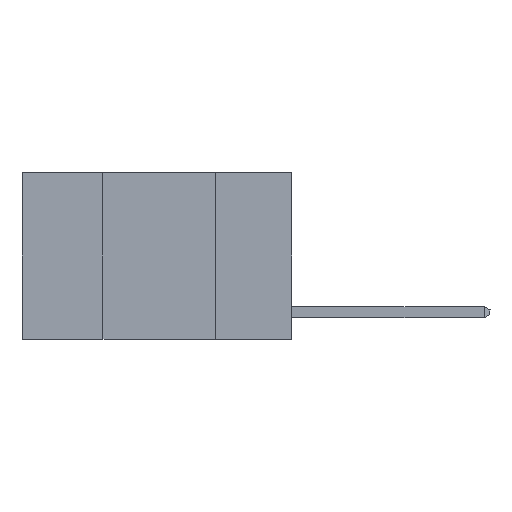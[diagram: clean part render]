
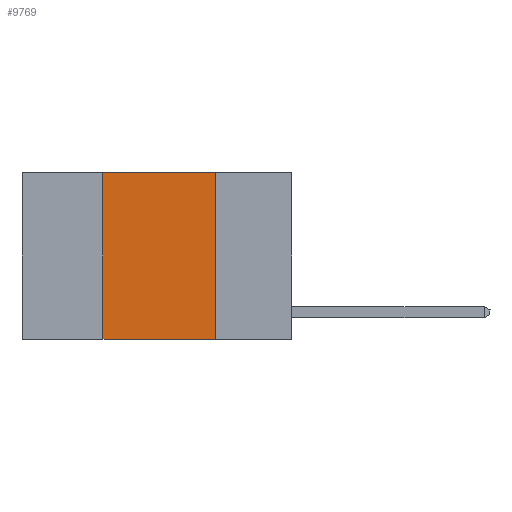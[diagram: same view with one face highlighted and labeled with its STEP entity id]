
A CAD part, left-side view. The second image highlights one B-rep face of the part: STEP entity #9769.
In plain terms, the highlighted planar face has unit normal (-1, 0, 0).
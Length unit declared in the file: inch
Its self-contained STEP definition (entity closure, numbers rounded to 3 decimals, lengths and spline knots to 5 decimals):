
#273 = LINE ( 'NONE', #14539, #352 ) ;
#352 = VECTOR ( 'NONE', #3297, 39.37008 ) ;
#1255 = ORIENTED_EDGE ( 'NONE', *, *, #9447, .F. ) ;
#1514 = VECTOR ( 'NONE', #4115, 39.37008 ) ;
#1585 = VERTEX_POINT ( 'NONE', #7413 ) ;
#3297 = DIRECTION ( 'NONE',  ( 0., -1., 0. ) ) ;
#3979 = DIRECTION ( 'NONE',  ( 0., 0., -1. ) ) ;
#3998 = LINE ( 'NONE', #9761, #4417 ) ;
#4010 = EDGE_CURVE ( 'NONE', #11095, #1585, #3998, .T. ) ;
#4115 = DIRECTION ( 'NONE',  ( 0., 0., -1. ) ) ;
#4417 = VECTOR ( 'NONE', #17045, 39.37008 ) ;
#4637 = CARTESIAN_POINT ( 'NONE',  ( 0., 0.17, 0. ) ) ;
#6352 = ORIENTED_EDGE ( 'NONE', *, *, #10274, .F. ) ;
#6619 = FACE_OUTER_BOUND ( 'NONE', #9994, .T. ) ;
#6963 = CARTESIAN_POINT ( 'NONE',  ( 0., 0.6, 0. ) ) ;
#7044 = VERTEX_POINT ( 'NONE', #4637 ) ;
#7413 = CARTESIAN_POINT ( 'NONE',  ( 0., 0.42, 0. ) ) ;
#9277 = ORIENTED_EDGE ( 'NONE', *, *, #11751, .T. ) ;
#9346 = VECTOR ( 'NONE', #15649, 39.37008 ) ;
#9447 = EDGE_CURVE ( 'NONE', #7044, #15120, #12897, .T. ) ;
#9761 = CARTESIAN_POINT ( 'NONE',  ( 0., 0.42, 0. ) ) ;
#9769 = ADVANCED_FACE ( 'NONE', ( #6619 ), #18179, .F. ) ;
#9894 = LINE ( 'NONE', #6963, #9346 ) ;
#9994 = EDGE_LOOP ( 'NONE', ( #1255, #6352, #14163, #9277 ) ) ;
#10274 = EDGE_CURVE ( 'NONE', #1585, #7044, #9894, .T. ) ;
#11095 = VERTEX_POINT ( 'NONE', #17304 ) ;
#11188 = CARTESIAN_POINT ( 'NONE',  ( 0., 0.17, 0. ) ) ;
#11751 = EDGE_CURVE ( 'NONE', #11095, #15120, #273, .T. ) ;
#12897 = LINE ( 'NONE', #11188, #1514 ) ;
#14163 = ORIENTED_EDGE ( 'NONE', *, *, #4010, .F. ) ;
#14539 = CARTESIAN_POINT ( 'NONE',  ( 0., 0.6, -0.37 ) ) ;
#15120 = VERTEX_POINT ( 'NONE', #15551 ) ;
#15404 = DIRECTION ( 'NONE',  ( 1., 0., 0. ) ) ;
#15551 = CARTESIAN_POINT ( 'NONE',  ( 0., 0.17, -0.37 ) ) ;
#15649 = DIRECTION ( 'NONE',  ( 0., -1., 0. ) ) ;
#16007 = AXIS2_PLACEMENT_3D ( 'NONE', #18358, #15404, #3979 ) ;
#17045 = DIRECTION ( 'NONE',  ( 0., 0., 1. ) ) ;
#17304 = CARTESIAN_POINT ( 'NONE',  ( 0., 0.42, -0.37 ) ) ;
#18179 = PLANE ( 'NONE',  #16007 ) ;
#18358 = CARTESIAN_POINT ( 'NONE',  ( 0., 0.6, 0. ) ) ;
